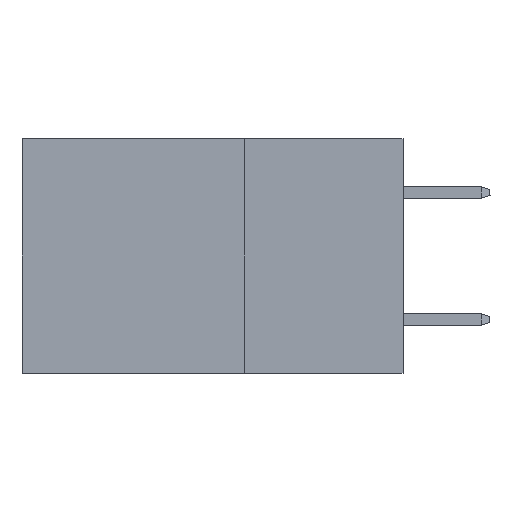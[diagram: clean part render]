
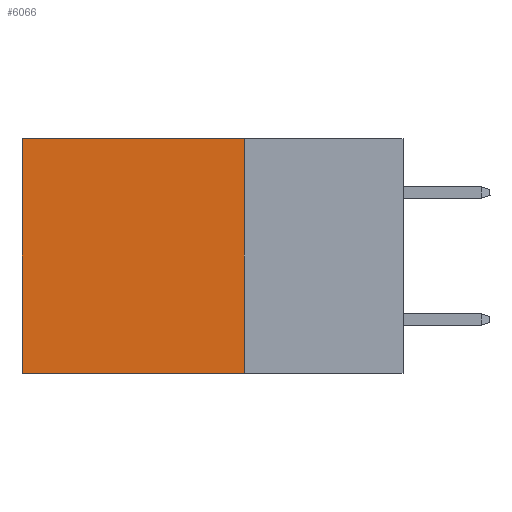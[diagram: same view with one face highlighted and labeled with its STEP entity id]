
A CAD part, left-side view. The second image highlights one B-rep face of the part: STEP entity #6066.
In plain terms, the highlighted planar face has unit normal (-1, 0, 0).
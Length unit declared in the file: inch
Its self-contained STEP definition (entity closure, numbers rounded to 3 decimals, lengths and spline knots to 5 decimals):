
#1183 = DIRECTION ( 'NONE',  ( 1., 0., 0. ) ) ;
#4006 = VECTOR ( 'NONE', #20502, 39.37008 ) ;
#4577 = VERTEX_POINT ( 'NONE', #9724 ) ;
#6066 = ADVANCED_FACE ( 'NONE', ( #30439 ), #40661, .F. ) ;
#9410 = CARTESIAN_POINT ( 'NONE',  ( 0.2875, 0.25, 0. ) ) ;
#9724 = CARTESIAN_POINT ( 'NONE',  ( 0.2875, 0.25, 0. ) ) ;
#10956 = EDGE_LOOP ( 'NONE', ( #27183, #18051, #18526, #20215 ) ) ;
#13256 = CARTESIAN_POINT ( 'NONE',  ( 0.2875, 0.25, -0.37 ) ) ;
#13510 = EDGE_CURVE ( 'NONE', #4577, #25076, #20113, .T. ) ;
#14177 = DIRECTION ( 'NONE',  ( 0., 0., -1. ) ) ;
#14322 = DIRECTION ( 'NONE',  ( 0., 1., 0. ) ) ;
#16778 = EDGE_CURVE ( 'NONE', #28997, #26256, #27361, .T. ) ;
#16843 = DIRECTION ( 'NONE',  ( 0., 0., -1. ) ) ;
#17743 = DIRECTION ( 'NONE',  ( 0., 1., 0. ) ) ;
#18051 = ORIENTED_EDGE ( 'NONE', *, *, #16778, .F. ) ;
#18526 = ORIENTED_EDGE ( 'NONE', *, *, #39033, .F. ) ;
#19508 = VECTOR ( 'NONE', #16843, 39.37008 ) ;
#20113 = LINE ( 'NONE', #33982, #23861 ) ;
#20215 = ORIENTED_EDGE ( 'NONE', *, *, #13510, .T. ) ;
#20502 = DIRECTION ( 'NONE',  ( 0., 0., -1. ) ) ;
#22159 = EDGE_CURVE ( 'NONE', #25076, #26256, #24126, .T. ) ;
#23861 = VECTOR ( 'NONE', #17743, 39.37008 ) ;
#24126 = LINE ( 'NONE', #30327, #19508 ) ;
#24428 = CARTESIAN_POINT ( 'NONE',  ( 0.2875, 0.25, 0. ) ) ;
#25076 = VERTEX_POINT ( 'NONE', #35366 ) ;
#25661 = LINE ( 'NONE', #9410, #4006 ) ;
#26256 = VERTEX_POINT ( 'NONE', #30930 ) ;
#27183 = ORIENTED_EDGE ( 'NONE', *, *, #22159, .T. ) ;
#27361 = LINE ( 'NONE', #33779, #30869 ) ;
#28997 = VERTEX_POINT ( 'NONE', #13256 ) ;
#30327 = CARTESIAN_POINT ( 'NONE',  ( 0.2875, 0.6, 0. ) ) ;
#30439 = FACE_OUTER_BOUND ( 'NONE', #10956, .T. ) ;
#30869 = VECTOR ( 'NONE', #14322, 39.37008 ) ;
#30930 = CARTESIAN_POINT ( 'NONE',  ( 0.2875, 0.6, -0.37 ) ) ;
#30955 = AXIS2_PLACEMENT_3D ( 'NONE', #24428, #1183, #14177 ) ;
#33779 = CARTESIAN_POINT ( 'NONE',  ( 0.2875, 0.25, -0.37 ) ) ;
#33982 = CARTESIAN_POINT ( 'NONE',  ( 0.2875, 0.25, 0. ) ) ;
#35366 = CARTESIAN_POINT ( 'NONE',  ( 0.2875, 0.6, 0. ) ) ;
#39033 = EDGE_CURVE ( 'NONE', #4577, #28997, #25661, .T. ) ;
#40661 = PLANE ( 'NONE',  #30955 ) ;
